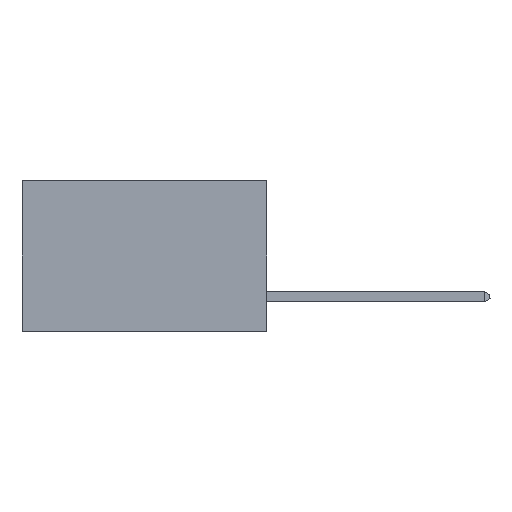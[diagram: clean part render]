
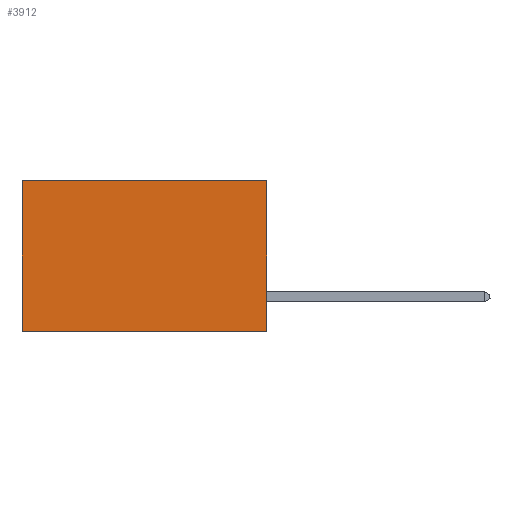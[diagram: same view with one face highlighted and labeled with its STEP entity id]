
A CAD part, left-side view. The second image highlights one B-rep face of the part: STEP entity #3912.
In plain terms, the highlighted planar face has unit normal (-1, 0, 0).
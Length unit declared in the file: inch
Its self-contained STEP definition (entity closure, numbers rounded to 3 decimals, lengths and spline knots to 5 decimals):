
#1671 = DIRECTION ( 'NONE',  ( 0., 1., 0. ) ) ;
#1898 = ORIENTED_EDGE ( 'NONE', *, *, #5442, .T. ) ;
#2035 = ORIENTED_EDGE ( 'NONE', *, *, #9912, .F. ) ;
#3912 = ADVANCED_FACE ( 'NONE', ( #4428 ), #16969, .F. ) ;
#4428 = FACE_OUTER_BOUND ( 'NONE', #17588, .T. ) ;
#5200 = VECTOR ( 'NONE', #1671, 39.37008 ) ;
#5218 = VERTEX_POINT ( 'NONE', #16683 ) ;
#5239 = CARTESIAN_POINT ( 'NONE',  ( 0.2875, 0.6, -0.37 ) ) ;
#5442 = EDGE_CURVE ( 'NONE', #17046, #8462, #8592, .T. ) ;
#6898 = DIRECTION ( 'NONE',  ( 0., 1., 0. ) ) ;
#7537 = EDGE_CURVE ( 'NONE', #16662, #5218, #14834, .T. ) ;
#7828 = CARTESIAN_POINT ( 'NONE',  ( 0.2875, 0., 0. ) ) ;
#8219 = EDGE_CURVE ( 'NONE', #16662, #17046, #15327, .T. ) ;
#8462 = VERTEX_POINT ( 'NONE', #5239 ) ;
#8592 = LINE ( 'NONE', #18822, #15943 ) ;
#9315 = AXIS2_PLACEMENT_3D ( 'NONE', #17111, #10648, #20319 ) ;
#9912 = EDGE_CURVE ( 'NONE', #5218, #8462, #10160, .T. ) ;
#10160 = LINE ( 'NONE', #14806, #13721 ) ;
#10648 = DIRECTION ( 'NONE',  ( 1., 0., 0. ) ) ;
#11021 = VECTOR ( 'NONE', #15553, 39.37008 ) ;
#11717 = CARTESIAN_POINT ( 'NONE',  ( 0.2875, 0., 0. ) ) ;
#13721 = VECTOR ( 'NONE', #6898, 39.37008 ) ;
#14091 = ORIENTED_EDGE ( 'NONE', *, *, #7537, .F. ) ;
#14806 = CARTESIAN_POINT ( 'NONE',  ( 0.2875, 0., -0.37 ) ) ;
#14834 = LINE ( 'NONE', #18691, #11021 ) ;
#15327 = LINE ( 'NONE', #7828, #5200 ) ;
#15553 = DIRECTION ( 'NONE',  ( 0., 0., -1. ) ) ;
#15943 = VECTOR ( 'NONE', #16237, 39.37008 ) ;
#16237 = DIRECTION ( 'NONE',  ( 0., 0., -1. ) ) ;
#16662 = VERTEX_POINT ( 'NONE', #11717 ) ;
#16683 = CARTESIAN_POINT ( 'NONE',  ( 0.2875, 0., -0.37 ) ) ;
#16969 = PLANE ( 'NONE',  #9315 ) ;
#17046 = VERTEX_POINT ( 'NONE', #17488 ) ;
#17111 = CARTESIAN_POINT ( 'NONE',  ( 0.2875, 0., 0. ) ) ;
#17488 = CARTESIAN_POINT ( 'NONE',  ( 0.2875, 0.6, 0. ) ) ;
#17588 = EDGE_LOOP ( 'NONE', ( #1898, #2035, #14091, #20013 ) ) ;
#18691 = CARTESIAN_POINT ( 'NONE',  ( 0.2875, 0., 0. ) ) ;
#18822 = CARTESIAN_POINT ( 'NONE',  ( 0.2875, 0.6, 0. ) ) ;
#20013 = ORIENTED_EDGE ( 'NONE', *, *, #8219, .T. ) ;
#20319 = DIRECTION ( 'NONE',  ( 0., 0., -1. ) ) ;
